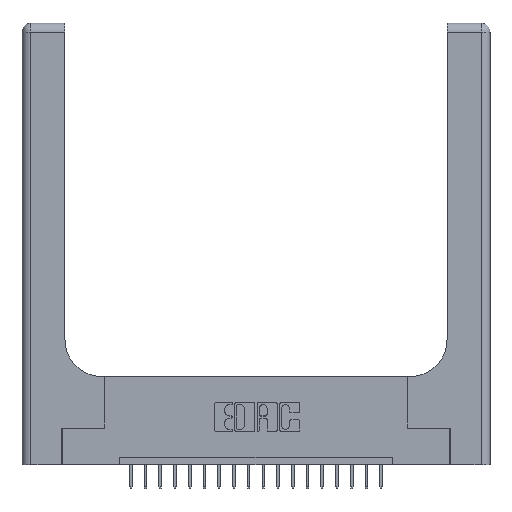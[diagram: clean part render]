
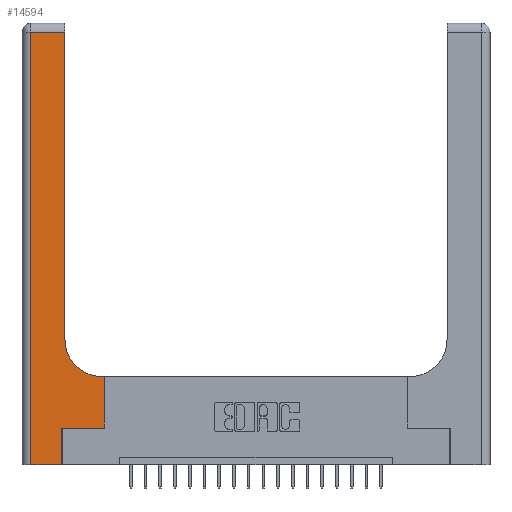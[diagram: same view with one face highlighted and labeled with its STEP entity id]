
A CAD part, top view. The second image highlights one B-rep face of the part: STEP entity #14594.
In plain terms, the highlighted planar face has unit normal (0, 0, 1).
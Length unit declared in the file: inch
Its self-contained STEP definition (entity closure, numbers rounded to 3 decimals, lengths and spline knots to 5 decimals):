
#132 = ORIENTED_EDGE ( 'NONE', *, *, #14050, .T. ) ;
#146 = VECTOR ( 'NONE', #20862, 39.37008 ) ;
#576 = VECTOR ( 'NONE', #11480, 39.37008 ) ;
#789 = LINE ( 'NONE', #21111, #21777 ) ;
#1079 = DIRECTION ( 'NONE',  ( 0., 0., -1. ) ) ;
#1160 = FACE_OUTER_BOUND ( 'NONE', #3177, .T. ) ;
#1556 = CARTESIAN_POINT ( 'NONE',  ( 0.5585, 0.25, 0.37 ) ) ;
#1764 = LINE ( 'NONE', #16417, #2828 ) ;
#2828 = VECTOR ( 'NONE', #16560, 39.37008 ) ;
#2851 = CARTESIAN_POINT ( 'NONE',  ( 0.5415, 0.6, 0.37 ) ) ;
#2987 = LINE ( 'NONE', #11027, #4831 ) ;
#3118 = CARTESIAN_POINT ( 'NONE',  ( 0.5415, 0.85, 0.37 ) ) ;
#3124 = EDGE_CURVE ( 'NONE', #17543, #5416, #16329, .T. ) ;
#3174 = ORIENTED_EDGE ( 'NONE', *, *, #9186, .T. ) ;
#3177 = EDGE_LOOP ( 'NONE', ( #12621, #3174, #6772, #14195, #19286, #21350, #15414, #5133, #132 ) ) ;
#4664 = LINE ( 'NONE', #20773, #146 ) ;
#4666 = VERTEX_POINT ( 'NONE', #2851 ) ;
#4824 = DIRECTION ( 'NONE',  ( 1., 0., 0. ) ) ;
#4831 = VECTOR ( 'NONE', #14600, 39.37008 ) ;
#5054 = VERTEX_POINT ( 'NONE', #16150 ) ;
#5133 = ORIENTED_EDGE ( 'NONE', *, *, #17069, .T. ) ;
#5168 = EDGE_CURVE ( 'NONE', #16762, #9276, #20443, .T. ) ;
#5416 = VERTEX_POINT ( 'NONE', #14542 ) ;
#5420 = EDGE_CURVE ( 'NONE', #9139, #5054, #789, .T. ) ;
#6163 = CARTESIAN_POINT ( 'NONE',  ( 0.2915, 3., 0.37 ) ) ;
#6772 = ORIENTED_EDGE ( 'NONE', *, *, #5420, .T. ) ;
#6936 = VERTEX_POINT ( 'NONE', #1556 ) ;
#6969 = AXIS2_PLACEMENT_3D ( 'NONE', #3118, #15081, #4824 ) ;
#7021 = CARTESIAN_POINT ( 'NONE',  ( 0.06, 2.94, 0.37 ) ) ;
#9139 = VERTEX_POINT ( 'NONE', #7021 ) ;
#9186 = EDGE_CURVE ( 'NONE', #5416, #9139, #19976, .T. ) ;
#9276 = VERTEX_POINT ( 'NONE', #17548 ) ;
#9714 = CIRCLE ( 'NONE', #6969, 0.25 ) ;
#10417 = AXIS2_PLACEMENT_3D ( 'NONE', #11296, #1079, #17442 ) ;
#11027 = CARTESIAN_POINT ( 'NONE',  ( 0.2915, 0.6, 0.37 ) ) ;
#11296 = CARTESIAN_POINT ( 'NONE',  ( 0., 3., 0.37 ) ) ;
#11480 = DIRECTION ( 'NONE',  ( 0., 1., 0. ) ) ;
#11575 = DIRECTION ( 'NONE',  ( 0., 1., 0. ) ) ;
#11830 = EDGE_CURVE ( 'NONE', #5054, #16762, #1764, .T. ) ;
#11990 = VECTOR ( 'NONE', #20541, 39.37008 ) ;
#12621 = ORIENTED_EDGE ( 'NONE', *, *, #3124, .T. ) ;
#13324 = EDGE_CURVE ( 'NONE', #6936, #18803, #16631, .T. ) ;
#13615 = CARTESIAN_POINT ( 'NONE',  ( 0., 2.94, 0.37 ) ) ;
#14050 = EDGE_CURVE ( 'NONE', #4666, #17543, #9714, .T. ) ;
#14195 = ORIENTED_EDGE ( 'NONE', *, *, #11830, .T. ) ;
#14542 = CARTESIAN_POINT ( 'NONE',  ( 0.2915, 2.94, 0.37 ) ) ;
#14594 = ADVANCED_FACE ( 'NONE', ( #1160 ), #19721, .F. ) ;
#14600 = DIRECTION ( 'NONE',  ( -1., 0., 0. ) ) ;
#15081 = DIRECTION ( 'NONE',  ( 0., 0., -1. ) ) ;
#15266 = EDGE_CURVE ( 'NONE', #9276, #6936, #4664, .T. ) ;
#15414 = ORIENTED_EDGE ( 'NONE', *, *, #13324, .T. ) ;
#15466 = CARTESIAN_POINT ( 'NONE',  ( 0.2915, 0.85, 0.37 ) ) ;
#16150 = CARTESIAN_POINT ( 'NONE',  ( 0.06, 0., 0.37 ) ) ;
#16329 = LINE ( 'NONE', #6163, #576 ) ;
#16417 = CARTESIAN_POINT ( 'NONE',  ( 0., 0., 0.37 ) ) ;
#16560 = DIRECTION ( 'NONE',  ( 1., 0., 0. ) ) ;
#16631 = LINE ( 'NONE', #18611, #21108 ) ;
#16762 = VERTEX_POINT ( 'NONE', #20073 ) ;
#17069 = EDGE_CURVE ( 'NONE', #18803, #4666, #2987, .T. ) ;
#17442 = DIRECTION ( 'NONE',  ( -1., 0., 0. ) ) ;
#17543 = VERTEX_POINT ( 'NONE', #15466 ) ;
#17548 = CARTESIAN_POINT ( 'NONE',  ( 0.269, 0.25, 0.37 ) ) ;
#18611 = CARTESIAN_POINT ( 'NONE',  ( 0.5585, 0.25, 0.37 ) ) ;
#18793 = CARTESIAN_POINT ( 'NONE',  ( 0.269, 0., 0.37 ) ) ;
#18803 = VERTEX_POINT ( 'NONE', #19324 ) ;
#19286 = ORIENTED_EDGE ( 'NONE', *, *, #5168, .T. ) ;
#19324 = CARTESIAN_POINT ( 'NONE',  ( 0.5585, 0.6, 0.37 ) ) ;
#19686 = DIRECTION ( 'NONE',  ( 0., -1., 0. ) ) ;
#19721 = PLANE ( 'NONE',  #10417 ) ;
#19976 = LINE ( 'NONE', #13615, #21042 ) ;
#20073 = CARTESIAN_POINT ( 'NONE',  ( 0.269, 0., 0.37 ) ) ;
#20443 = LINE ( 'NONE', #18793, #11990 ) ;
#20541 = DIRECTION ( 'NONE',  ( 0., 1., 0. ) ) ;
#20770 = DIRECTION ( 'NONE',  ( -1., 0., 0. ) ) ;
#20773 = CARTESIAN_POINT ( 'NONE',  ( 0.269, 0.25, 0.37 ) ) ;
#20862 = DIRECTION ( 'NONE',  ( 1., 0., 0. ) ) ;
#21042 = VECTOR ( 'NONE', #20770, 39.37008 ) ;
#21108 = VECTOR ( 'NONE', #11575, 39.37008 ) ;
#21111 = CARTESIAN_POINT ( 'NONE',  ( 0.06, 3., 0.37 ) ) ;
#21350 = ORIENTED_EDGE ( 'NONE', *, *, #15266, .T. ) ;
#21777 = VECTOR ( 'NONE', #19686, 39.37008 ) ;
